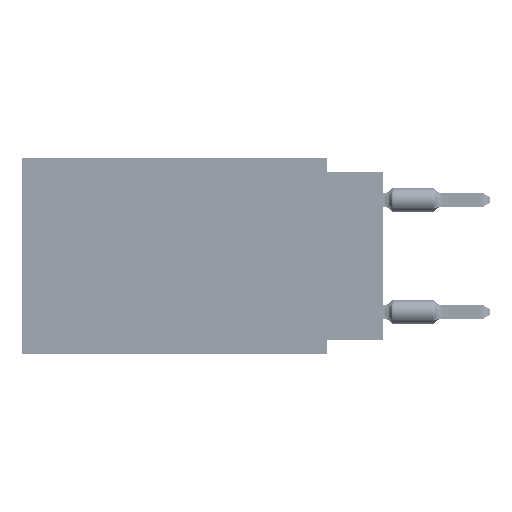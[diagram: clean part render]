
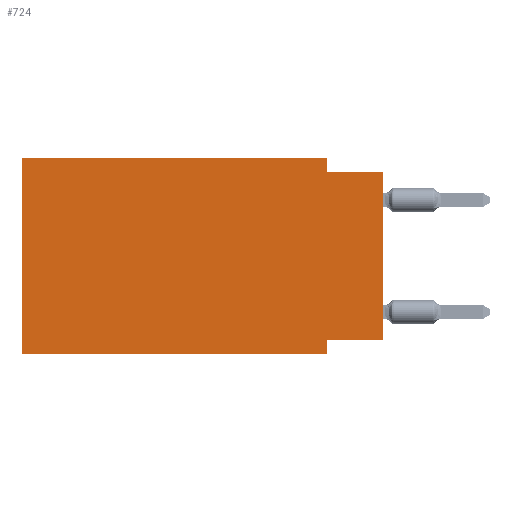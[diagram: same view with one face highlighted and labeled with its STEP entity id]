
A CAD part, left-side view. The second image highlights one B-rep face of the part: STEP entity #724.
In plain terms, the highlighted planar face has unit normal (-1, 0, 0).
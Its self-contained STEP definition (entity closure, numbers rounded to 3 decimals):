
#339 = EDGE_CURVE ( 'NONE', #42550, #55041, #43441, .T. ) ;
#724 = ADVANCED_FACE ( 'NONE', ( #33669 ), #22923, .F. ) ;
#1159 = VERTEX_POINT ( 'NONE', #54713 ) ;
#2071 = CARTESIAN_POINT ( 'NONE',  ( 0., 16.383, 0. ) ) ;
#4701 = ORIENTED_EDGE ( 'NONE', *, *, #44101, .F. ) ;
#4886 = CARTESIAN_POINT ( 'NONE',  ( 0., 2.54, -8.89 ) ) ;
#5271 = ORIENTED_EDGE ( 'NONE', *, *, #7585, .F. ) ;
#5345 = DIRECTION ( 'NONE',  ( 0., 0., -1. ) ) ;
#5542 = LINE ( 'NONE', #27432, #23888 ) ;
#6480 = LINE ( 'NONE', #50195, #60544 ) ;
#7585 = EDGE_CURVE ( 'NONE', #42550, #45513, #6480, .T. ) ;
#8210 = DIRECTION ( 'NONE',  ( 0., 1., 0. ) ) ;
#9647 = CARTESIAN_POINT ( 'NONE',  ( 0., 0., -0.635 ) ) ;
#11304 = LINE ( 'NONE', #22433, #32387 ) ;
#11305 = VECTOR ( 'NONE', #52112, 1000. ) ;
#11562 = ORIENTED_EDGE ( 'NONE', *, *, #17245, .F. ) ;
#14641 = CARTESIAN_POINT ( 'NONE',  ( 0., 0., -8.255 ) ) ;
#17245 = EDGE_CURVE ( 'NONE', #62860, #45452, #18975, .T. ) ;
#18975 = LINE ( 'NONE', #14641, #32273 ) ;
#19261 = DIRECTION ( 'NONE',  ( 0., -1., 0. ) ) ;
#19610 = LINE ( 'NONE', #2071, #30201 ) ;
#19716 = LINE ( 'NONE', #9647, #25587 ) ;
#22433 = CARTESIAN_POINT ( 'NONE',  ( 0., 2.54, -8.89 ) ) ;
#22850 = CARTESIAN_POINT ( 'NONE',  ( 0., 0., -0.635 ) ) ;
#22923 = PLANE ( 'NONE',  #52996 ) ;
#23440 = ORIENTED_EDGE ( 'NONE', *, *, #55729, .F. ) ;
#23888 = VECTOR ( 'NONE', #43538, 1000. ) ;
#25102 = ORIENTED_EDGE ( 'NONE', *, *, #57620, .F. ) ;
#25249 = LINE ( 'NONE', #52802, #11305 ) ;
#25587 = VECTOR ( 'NONE', #31547, 1000. ) ;
#27049 = CARTESIAN_POINT ( 'NONE',  ( 0., 16.383, 0. ) ) ;
#27432 = CARTESIAN_POINT ( 'NONE',  ( 0., 0., 0. ) ) ;
#28151 = DIRECTION ( 'NONE',  ( 0., 0., -1. ) ) ;
#30166 = VERTEX_POINT ( 'NONE', #22850 ) ;
#30201 = VECTOR ( 'NONE', #19261, 1000. ) ;
#31547 = DIRECTION ( 'NONE',  ( 0., -1., 0. ) ) ;
#31718 = ORIENTED_EDGE ( 'NONE', *, *, #50188, .T. ) ;
#32273 = VECTOR ( 'NONE', #8210, 1000. ) ;
#32387 = VECTOR ( 'NONE', #28151, 1000. ) ;
#32399 = ORIENTED_EDGE ( 'NONE', *, *, #339, .T. ) ;
#33669 = FACE_OUTER_BOUND ( 'NONE', #51585, .T. ) ;
#33946 = CARTESIAN_POINT ( 'NONE',  ( 0., 2.54, -0.635 ) ) ;
#38772 = CARTESIAN_POINT ( 'NONE',  ( 0., 16.383, -8.89 ) ) ;
#42088 = CARTESIAN_POINT ( 'NONE',  ( 0., 2.54, -8.255 ) ) ;
#42550 = VERTEX_POINT ( 'NONE', #65700 ) ;
#43441 = LINE ( 'NONE', #38772, #70126 ) ;
#43538 = DIRECTION ( 'NONE',  ( 0., 0., 1. ) ) ;
#43700 = CARTESIAN_POINT ( 'NONE',  ( 0., 16.383, 0. ) ) ;
#44101 = EDGE_CURVE ( 'NONE', #1159, #49812, #25249, .T. ) ;
#44494 = DIRECTION ( 'NONE',  ( 0., -1., 0. ) ) ;
#45452 = VERTEX_POINT ( 'NONE', #42088 ) ;
#45513 = VERTEX_POINT ( 'NONE', #27049 ) ;
#48120 = CARTESIAN_POINT ( 'NONE',  ( 0., 0., -8.255 ) ) ;
#49812 = VERTEX_POINT ( 'NONE', #33946 ) ;
#50188 = EDGE_CURVE ( 'NONE', #62860, #30166, #5542, .T. ) ;
#50195 = CARTESIAN_POINT ( 'NONE',  ( 0., 16.383, 0. ) ) ;
#51585 = EDGE_LOOP ( 'NONE', ( #31718, #23440, #4701, #25102, #5271, #32399, #61433, #11562 ) ) ;
#52112 = DIRECTION ( 'NONE',  ( 0., 0., -1. ) ) ;
#52802 = CARTESIAN_POINT ( 'NONE',  ( 0., 2.54, 0. ) ) ;
#52996 = AXIS2_PLACEMENT_3D ( 'NONE', #43700, #55485, #5345 ) ;
#54713 = CARTESIAN_POINT ( 'NONE',  ( 0., 2.54, 0. ) ) ;
#55041 = VERTEX_POINT ( 'NONE', #4886 ) ;
#55485 = DIRECTION ( 'NONE',  ( 1., 0., 0. ) ) ;
#55729 = EDGE_CURVE ( 'NONE', #49812, #30166, #19716, .T. ) ;
#57620 = EDGE_CURVE ( 'NONE', #45513, #1159, #19610, .T. ) ;
#60544 = VECTOR ( 'NONE', #61270, 1000. ) ;
#61270 = DIRECTION ( 'NONE',  ( 0., 0., 1. ) ) ;
#61433 = ORIENTED_EDGE ( 'NONE', *, *, #62586, .F. ) ;
#62586 = EDGE_CURVE ( 'NONE', #45452, #55041, #11304, .T. ) ;
#62860 = VERTEX_POINT ( 'NONE', #48120 ) ;
#65700 = CARTESIAN_POINT ( 'NONE',  ( 0., 16.383, -8.89 ) ) ;
#70126 = VECTOR ( 'NONE', #44494, 1000. ) ;
